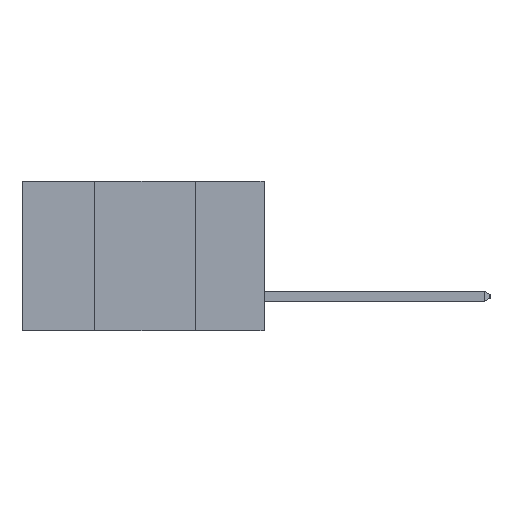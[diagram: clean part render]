
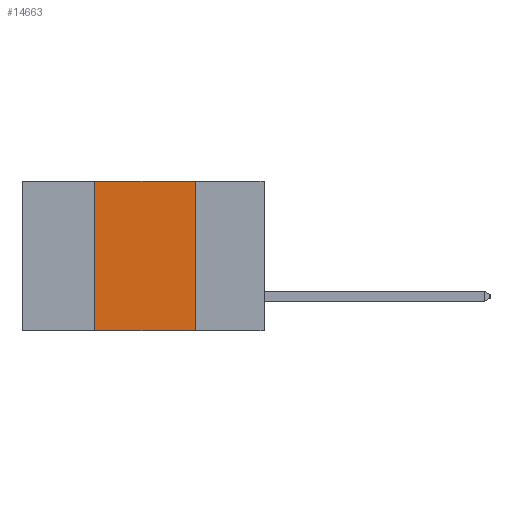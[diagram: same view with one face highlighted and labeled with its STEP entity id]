
A CAD part, left-side view. The second image highlights one B-rep face of the part: STEP entity #14663.
In plain terms, the highlighted planar face has unit normal (-1, 0, 0).
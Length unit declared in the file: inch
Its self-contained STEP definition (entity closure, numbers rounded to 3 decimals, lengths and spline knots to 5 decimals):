
#363 = LINE ( 'NONE', #5703, #18537 ) ;
#935 = CARTESIAN_POINT ( 'NONE',  ( 0., 0.6, 0. ) ) ;
#1228 = VERTEX_POINT ( 'NONE', #10977 ) ;
#1623 = EDGE_LOOP ( 'NONE', ( #12853, #2633, #4138, #18255 ) ) ;
#2535 = LINE ( 'NONE', #14751, #10921 ) ;
#2633 = ORIENTED_EDGE ( 'NONE', *, *, #13683, .F. ) ;
#3070 = VECTOR ( 'NONE', #18009, 39.37008 ) ;
#3507 = DIRECTION ( 'NONE',  ( 0., 0., -1. ) ) ;
#3760 = VERTEX_POINT ( 'NONE', #9800 ) ;
#4138 = ORIENTED_EDGE ( 'NONE', *, *, #11663, .F. ) ;
#4263 = EDGE_CURVE ( 'NONE', #3760, #7769, #363, .T. ) ;
#5343 = DIRECTION ( 'NONE',  ( 0., 0., -1. ) ) ;
#5703 = CARTESIAN_POINT ( 'NONE',  ( 0., 0.17, -0.37 ) ) ;
#6738 = FACE_OUTER_BOUND ( 'NONE', #1623, .T. ) ;
#7769 = VERTEX_POINT ( 'NONE', #14100 ) ;
#9017 = VERTEX_POINT ( 'NONE', #17545 ) ;
#9800 = CARTESIAN_POINT ( 'NONE',  ( 0., 0.17, 0. ) ) ;
#10251 = VECTOR ( 'NONE', #15134, 39.37008 ) ;
#10921 = VECTOR ( 'NONE', #14676, 39.37008 ) ;
#10977 = CARTESIAN_POINT ( 'NONE',  ( 0., 0.42, -0.37 ) ) ;
#11354 = EDGE_CURVE ( 'NONE', #1228, #7769, #21468, .T. ) ;
#11663 = EDGE_CURVE ( 'NONE', #1228, #9017, #2535, .T. ) ;
#12853 = ORIENTED_EDGE ( 'NONE', *, *, #4263, .F. ) ;
#13683 = EDGE_CURVE ( 'NONE', #9017, #3760, #14906, .T. ) ;
#14100 = CARTESIAN_POINT ( 'NONE',  ( 0., 0.17, -0.37 ) ) ;
#14117 = DIRECTION ( 'NONE',  ( 1., 0., 0. ) ) ;
#14663 = ADVANCED_FACE ( 'NONE', ( #6738 ), #20760, .F. ) ;
#14676 = DIRECTION ( 'NONE',  ( 0., 0., 1. ) ) ;
#14751 = CARTESIAN_POINT ( 'NONE',  ( 0., 0.42, -0.37 ) ) ;
#14906 = LINE ( 'NONE', #935, #10251 ) ;
#15134 = DIRECTION ( 'NONE',  ( 0., -1., 0. ) ) ;
#17434 = CARTESIAN_POINT ( 'NONE',  ( 0., 0.6, 0. ) ) ;
#17545 = CARTESIAN_POINT ( 'NONE',  ( 0., 0.42, 0. ) ) ;
#17600 = AXIS2_PLACEMENT_3D ( 'NONE', #17434, #14117, #3507 ) ;
#18009 = DIRECTION ( 'NONE',  ( 0., -1., 0. ) ) ;
#18255 = ORIENTED_EDGE ( 'NONE', *, *, #11354, .T. ) ;
#18456 = CARTESIAN_POINT ( 'NONE',  ( 0., 0.6, -0.37 ) ) ;
#18537 = VECTOR ( 'NONE', #5343, 39.37008 ) ;
#20760 = PLANE ( 'NONE',  #17600 ) ;
#21468 = LINE ( 'NONE', #18456, #3070 ) ;
